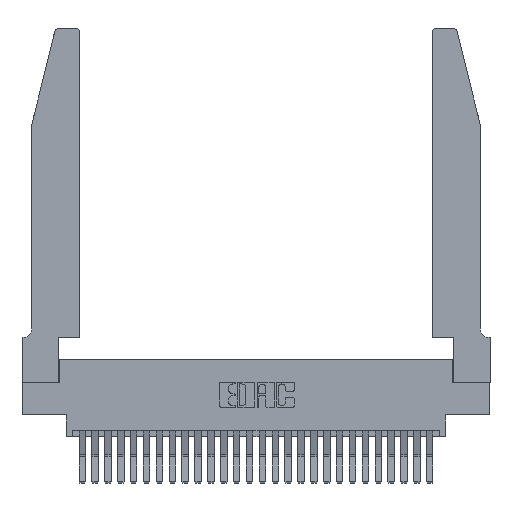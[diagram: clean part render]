
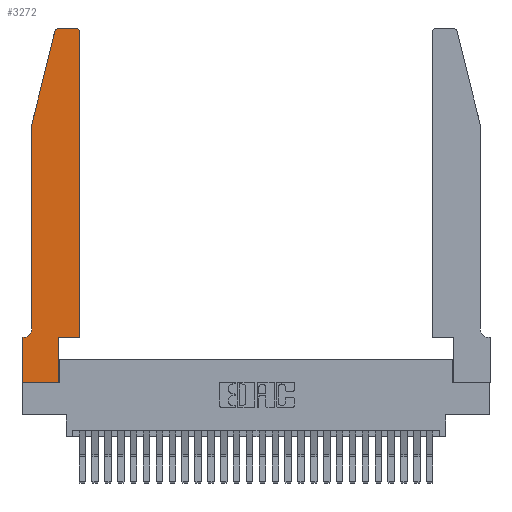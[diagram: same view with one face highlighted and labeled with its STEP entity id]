
A CAD part, top view. The second image highlights one B-rep face of the part: STEP entity #3272.
In plain terms, the highlighted planar face has unit normal (0, 0, 1).
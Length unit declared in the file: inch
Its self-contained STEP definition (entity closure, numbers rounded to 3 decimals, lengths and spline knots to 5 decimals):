
#258 = VECTOR ( 'NONE', #8307, 39.37008 ) ;
#323 = ORIENTED_EDGE ( 'NONE', *, *, #11660, .T. ) ;
#605 = CARTESIAN_POINT ( 'NONE',  ( 0.2865, 0., 0.37 ) ) ;
#646 = EDGE_CURVE ( 'NONE', #18790, #22317, #17849, .T. ) ;
#703 = FACE_OUTER_BOUND ( 'NONE', #12808, .T. ) ;
#951 = LINE ( 'NONE', #12483, #23997 ) ;
#1075 = VERTEX_POINT ( 'NONE', #10910 ) ;
#1107 = ORIENTED_EDGE ( 'NONE', *, *, #25023, .T. ) ;
#1315 = CIRCLE ( 'NONE', #21970, 0.03 ) ;
#1534 = DIRECTION ( 'NONE',  ( 0., -1., 0. ) ) ;
#1555 = CARTESIAN_POINT ( 'NONE',  ( 0.4505, 2.72, 0.37 ) ) ;
#1632 = VERTEX_POINT ( 'NONE', #605 ) ;
#1682 = VERTEX_POINT ( 'NONE', #18074 ) ;
#1709 = ORIENTED_EDGE ( 'NONE', *, *, #27398, .T. ) ;
#1933 = VECTOR ( 'NONE', #22444, 39.37008 ) ;
#1994 = CARTESIAN_POINT ( 'NONE',  ( 0.284, 2.72, 0.37 ) ) ;
#2268 = ORIENTED_EDGE ( 'NONE', *, *, #15087, .T. ) ;
#2781 = AXIS2_PLACEMENT_3D ( 'NONE', #3321, #19086, #5592 ) ;
#3054 = CARTESIAN_POINT ( 'NONE',  ( 0.0755, 2., 0.37 ) ) ;
#3272 = ADVANCED_FACE ( 'NONE', ( #703 ), #27695, .T. ) ;
#3321 = CARTESIAN_POINT ( 'NONE',  ( 0., 0.35, 0.37 ) ) ;
#3803 = DIRECTION ( 'NONE',  ( 1., 0., 0. ) ) ;
#4285 = DIRECTION ( 'NONE',  ( 1., 0., 0. ) ) ;
#4586 = EDGE_CURVE ( 'NONE', #11293, #1075, #9934, .T. ) ;
#4738 = CARTESIAN_POINT ( 'NONE',  ( 0.284, 2.75, 0.37 ) ) ;
#5592 = DIRECTION ( 'NONE',  ( 1., 0., 0. ) ) ;
#5839 = LINE ( 'NONE', #12752, #17162 ) ;
#5862 = ORIENTED_EDGE ( 'NONE', *, *, #7269, .T. ) ;
#5944 = DIRECTION ( 'NONE',  ( 1., 0., 0. ) ) ;
#6017 = CARTESIAN_POINT ( 'NONE',  ( 0.0755, 2., 0.37 ) ) ;
#7269 = EDGE_CURVE ( 'NONE', #1682, #1632, #12648, .T. ) ;
#7755 = VERTEX_POINT ( 'NONE', #3054 ) ;
#8307 = DIRECTION ( 'NONE',  ( -0.239, -0.971, 0. ) ) ;
#9179 = ORIENTED_EDGE ( 'NONE', *, *, #26729, .T. ) ;
#9305 = AXIS2_PLACEMENT_3D ( 'NONE', #9458, #24888, #11784 ) ;
#9306 = VERTEX_POINT ( 'NONE', #22125 ) ;
#9458 = CARTESIAN_POINT ( 'NONE',  ( 0.4205, 2.72, 0.37 ) ) ;
#9719 = DIRECTION ( 'NONE',  ( 0., 1., 0. ) ) ;
#9934 = LINE ( 'NONE', #25807, #26822 ) ;
#10459 = CARTESIAN_POINT ( 'NONE',  ( 0.0755, 0.42, 0.37 ) ) ;
#10766 = DIRECTION ( 'NONE',  ( 0., 0., -1. ) ) ;
#10910 = CARTESIAN_POINT ( 'NONE',  ( 0., 0.35, 0.37 ) ) ;
#11293 = VERTEX_POINT ( 'NONE', #18421 ) ;
#11660 = EDGE_CURVE ( 'NONE', #1632, #20149, #16266, .T. ) ;
#11784 = DIRECTION ( 'NONE',  ( 1., 0., 0. ) ) ;
#12185 = CARTESIAN_POINT ( 'NONE',  ( 0.2865, 0.35, 0.37 ) ) ;
#12368 = LINE ( 'NONE', #6017, #258 ) ;
#12470 = EDGE_CURVE ( 'NONE', #7755, #27843, #951, .T. ) ;
#12483 = CARTESIAN_POINT ( 'NONE',  ( 0.0755, 2., 0.37 ) ) ;
#12648 = LINE ( 'NONE', #21592, #28754 ) ;
#12671 = VECTOR ( 'NONE', #3803, 39.37008 ) ;
#12752 = CARTESIAN_POINT ( 'NONE',  ( 0.2605, 2.75, 0.37 ) ) ;
#12808 = EDGE_LOOP ( 'NONE', ( #26625, #1107, #9179, #20731, #28763, #23864, #23587, #5862, #323, #1709, #13109, #2268 ) ) ;
#13109 = ORIENTED_EDGE ( 'NONE', *, *, #646, .T. ) ;
#13411 = VECTOR ( 'NONE', #20252, 39.37008 ) ;
#14138 = VERTEX_POINT ( 'NONE', #4738 ) ;
#14968 = DIRECTION ( 'NONE',  ( -1., 0., 0. ) ) ;
#15010 = CARTESIAN_POINT ( 'NONE',  ( 0.2865, 0.35, 0.37 ) ) ;
#15087 = EDGE_CURVE ( 'NONE', #22317, #24296, #26066, .T. ) ;
#15439 = EDGE_CURVE ( 'NONE', #27843, #11293, #22337, .T. ) ;
#16266 = LINE ( 'NONE', #15010, #27119 ) ;
#17162 = VECTOR ( 'NONE', #28077, 39.37008 ) ;
#17811 = DIRECTION ( 'NONE',  ( 0., 0., 1. ) ) ;
#17849 = LINE ( 'NONE', #20720, #1933 ) ;
#18056 = CARTESIAN_POINT ( 'NONE',  ( 0., 0., 0.37 ) ) ;
#18074 = CARTESIAN_POINT ( 'NONE',  ( 0., 0., 0.37 ) ) ;
#18421 = CARTESIAN_POINT ( 'NONE',  ( 0.0055, 0.35, 0.37 ) ) ;
#18790 = VERTEX_POINT ( 'NONE', #22825 ) ;
#19086 = DIRECTION ( 'NONE',  ( 0., 0., 1. ) ) ;
#19860 = CARTESIAN_POINT ( 'NONE',  ( 0.4205, 2.75, 0.37 ) ) ;
#20149 = VERTEX_POINT ( 'NONE', #12185 ) ;
#20252 = DIRECTION ( 'NONE',  ( 0., -1., 0. ) ) ;
#20362 = EDGE_CURVE ( 'NONE', #24296, #14138, #5839, .T. ) ;
#20720 = CARTESIAN_POINT ( 'NONE',  ( 0.4505, 0.35, 0.37 ) ) ;
#20731 = ORIENTED_EDGE ( 'NONE', *, *, #12470, .T. ) ;
#21592 = CARTESIAN_POINT ( 'NONE',  ( 0., 0., 0.37 ) ) ;
#21970 = AXIS2_PLACEMENT_3D ( 'NONE', #1994, #17811, #4285 ) ;
#22125 = CARTESIAN_POINT ( 'NONE',  ( 0.25487, 2.72718, 0.37 ) ) ;
#22165 = AXIS2_PLACEMENT_3D ( 'NONE', #23934, #10766, #26136 ) ;
#22317 = VERTEX_POINT ( 'NONE', #1555 ) ;
#22337 = CIRCLE ( 'NONE', #22165, 0.07 ) ;
#22444 = DIRECTION ( 'NONE',  ( 0., 1., 0. ) ) ;
#22825 = CARTESIAN_POINT ( 'NONE',  ( 0.4505, 0.35, 0.37 ) ) ;
#23587 = ORIENTED_EDGE ( 'NONE', *, *, #26880, .T. ) ;
#23639 = LINE ( 'NONE', #28255, #12671 ) ;
#23864 = ORIENTED_EDGE ( 'NONE', *, *, #4586, .T. ) ;
#23934 = CARTESIAN_POINT ( 'NONE',  ( 0.0055, 0.42, 0.37 ) ) ;
#23997 = VECTOR ( 'NONE', #1534, 39.37008 ) ;
#24296 = VERTEX_POINT ( 'NONE', #19860 ) ;
#24888 = DIRECTION ( 'NONE',  ( 0., 0., 1. ) ) ;
#25010 = LINE ( 'NONE', #18056, #13411 ) ;
#25023 = EDGE_CURVE ( 'NONE', #14138, #9306, #1315, .T. ) ;
#25807 = CARTESIAN_POINT ( 'NONE',  ( 0.0755, 0.35, 0.37 ) ) ;
#26066 = CIRCLE ( 'NONE', #9305, 0.03 ) ;
#26136 = DIRECTION ( 'NONE',  ( -1., 0., 0. ) ) ;
#26625 = ORIENTED_EDGE ( 'NONE', *, *, #20362, .T. ) ;
#26729 = EDGE_CURVE ( 'NONE', #9306, #7755, #12368, .T. ) ;
#26822 = VECTOR ( 'NONE', #14968, 39.37008 ) ;
#26880 = EDGE_CURVE ( 'NONE', #1075, #1682, #25010, .T. ) ;
#27119 = VECTOR ( 'NONE', #9719, 39.37008 ) ;
#27398 = EDGE_CURVE ( 'NONE', #20149, #18790, #23639, .T. ) ;
#27695 = PLANE ( 'NONE',  #2781 ) ;
#27843 = VERTEX_POINT ( 'NONE', #10459 ) ;
#28077 = DIRECTION ( 'NONE',  ( -1., 0., 0. ) ) ;
#28255 = CARTESIAN_POINT ( 'NONE',  ( 0.4505, 0.35, 0.37 ) ) ;
#28754 = VECTOR ( 'NONE', #5944, 39.37008 ) ;
#28763 = ORIENTED_EDGE ( 'NONE', *, *, #15439, .T. ) ;
